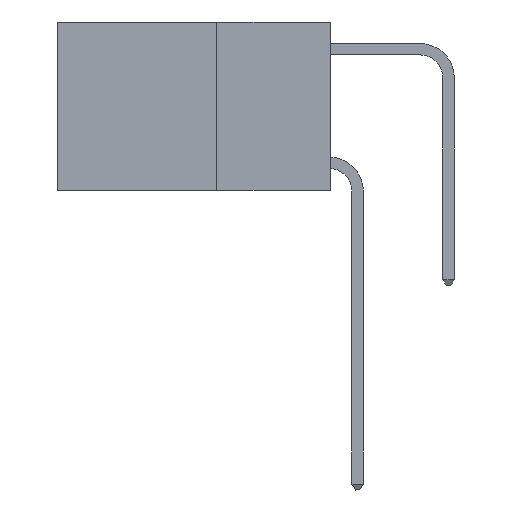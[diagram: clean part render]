
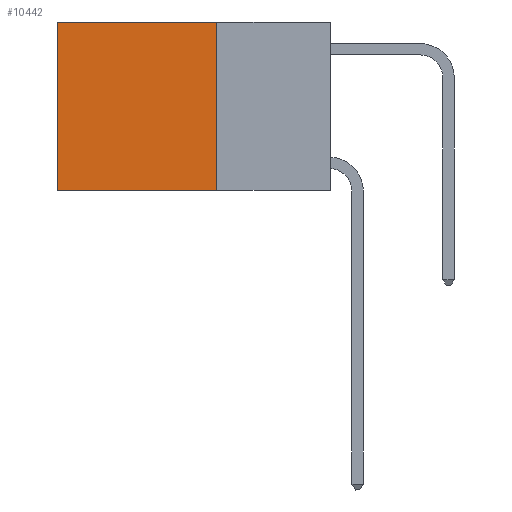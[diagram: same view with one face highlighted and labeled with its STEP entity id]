
A CAD part, left-side view. The second image highlights one B-rep face of the part: STEP entity #10442.
In plain terms, the highlighted planar face has unit normal (-1, 0, 0).
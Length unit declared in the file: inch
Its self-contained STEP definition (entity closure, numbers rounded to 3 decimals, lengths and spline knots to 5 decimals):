
#422 = CARTESIAN_POINT ( 'NONE',  ( 0.2625, 0.25, -0.37 ) ) ;
#725 = LINE ( 'NONE', #9039, #22238 ) ;
#1407 = ORIENTED_EDGE ( 'NONE', *, *, #2551, .T. ) ;
#1560 = DIRECTION ( 'NONE',  ( 0., 1., 0. ) ) ;
#2239 = VECTOR ( 'NONE', #6277, 39.37008 ) ;
#2551 = EDGE_CURVE ( 'NONE', #10073, #7251, #19927, .T. ) ;
#3529 = CARTESIAN_POINT ( 'NONE',  ( 0.2625, 0.25, 0. ) ) ;
#3758 = EDGE_CURVE ( 'NONE', #13128, #10073, #725, .T. ) ;
#4221 = CARTESIAN_POINT ( 'NONE',  ( 0.2625, 0.25, 0. ) ) ;
#5325 = DIRECTION ( 'NONE',  ( 1., 0., 0. ) ) ;
#5796 = CARTESIAN_POINT ( 'NONE',  ( 0.2625, 0.6, 0. ) ) ;
#6037 = VERTEX_POINT ( 'NONE', #422 ) ;
#6277 = DIRECTION ( 'NONE',  ( 0., 0., -1. ) ) ;
#6829 = CARTESIAN_POINT ( 'NONE',  ( 0.2625, 0.25, -0.37 ) ) ;
#7030 = DIRECTION ( 'NONE',  ( 0., 0., -1. ) ) ;
#7251 = VERTEX_POINT ( 'NONE', #10021 ) ;
#9039 = CARTESIAN_POINT ( 'NONE',  ( 0.2625, 0.25, 0. ) ) ;
#9587 = CARTESIAN_POINT ( 'NONE',  ( 0.2625, 0.6, 0. ) ) ;
#10021 = CARTESIAN_POINT ( 'NONE',  ( 0.2625, 0.6, -0.37 ) ) ;
#10073 = VERTEX_POINT ( 'NONE', #5796 ) ;
#10221 = EDGE_CURVE ( 'NONE', #13128, #6037, #19779, .T. ) ;
#10351 = ORIENTED_EDGE ( 'NONE', *, *, #15808, .F. ) ;
#10442 = ADVANCED_FACE ( 'NONE', ( #16112 ), #14160, .F. ) ;
#12733 = VECTOR ( 'NONE', #14642, 39.37008 ) ;
#12858 = ORIENTED_EDGE ( 'NONE', *, *, #10221, .F. ) ;
#13128 = VERTEX_POINT ( 'NONE', #19493 ) ;
#14160 = PLANE ( 'NONE',  #17862 ) ;
#14642 = DIRECTION ( 'NONE',  ( 0., 0., -1. ) ) ;
#15808 = EDGE_CURVE ( 'NONE', #6037, #7251, #19346, .T. ) ;
#15885 = ORIENTED_EDGE ( 'NONE', *, *, #3758, .T. ) ;
#16112 = FACE_OUTER_BOUND ( 'NONE', #16555, .T. ) ;
#16555 = EDGE_LOOP ( 'NONE', ( #1407, #10351, #12858, #15885 ) ) ;
#17756 = VECTOR ( 'NONE', #1560, 39.37008 ) ;
#17862 = AXIS2_PLACEMENT_3D ( 'NONE', #3529, #5325, #7030 ) ;
#19346 = LINE ( 'NONE', #6829, #17756 ) ;
#19493 = CARTESIAN_POINT ( 'NONE',  ( 0.2625, 0.25, 0. ) ) ;
#19779 = LINE ( 'NONE', #4221, #12733 ) ;
#19927 = LINE ( 'NONE', #9587, #2239 ) ;
#21362 = DIRECTION ( 'NONE',  ( 0., 1., 0. ) ) ;
#22238 = VECTOR ( 'NONE', #21362, 39.37008 ) ;
